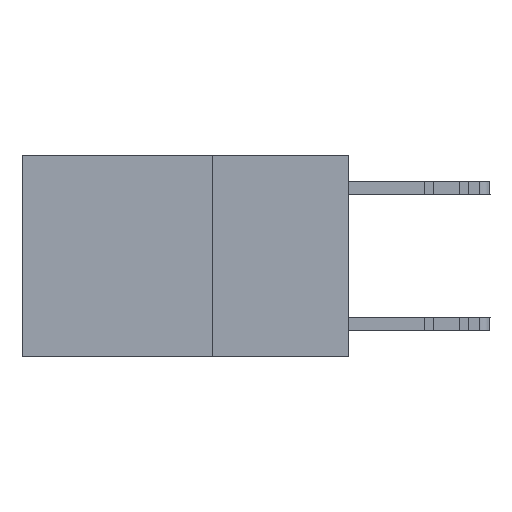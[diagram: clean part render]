
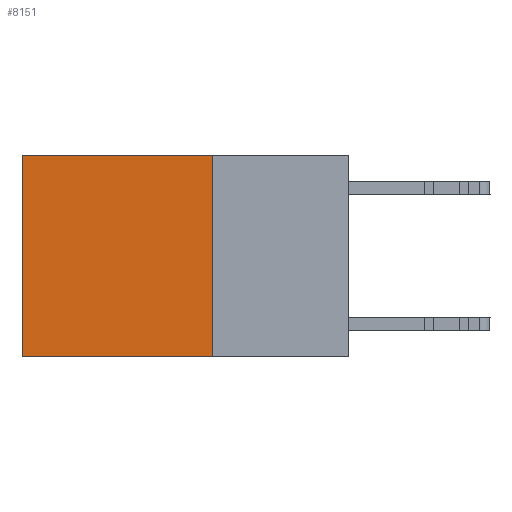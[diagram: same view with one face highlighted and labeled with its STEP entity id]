
A CAD part, left-side view. The second image highlights one B-rep face of the part: STEP entity #8151.
In plain terms, the highlighted planar face has unit normal (-1, 0, 0).
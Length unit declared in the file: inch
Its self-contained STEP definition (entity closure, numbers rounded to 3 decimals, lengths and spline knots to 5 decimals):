
#468 = ORIENTED_EDGE ( 'NONE', *, *, #17017, .T. ) ;
#473 = VECTOR ( 'NONE', #4716, 39.37008 ) ;
#1434 = LINE ( 'NONE', #5708, #473 ) ;
#2839 = CARTESIAN_POINT ( 'NONE',  ( 0.2625, 0.25, 0. ) ) ;
#3138 = DIRECTION ( 'NONE',  ( 0., 0., -1. ) ) ;
#3857 = VERTEX_POINT ( 'NONE', #8000 ) ;
#3904 = EDGE_CURVE ( 'NONE', #3857, #25204, #1434, .T. ) ;
#4211 = EDGE_LOOP ( 'NONE', ( #19752, #15966, #17215, #468 ) ) ;
#4716 = DIRECTION ( 'NONE',  ( 0., 0., -1. ) ) ;
#5372 = DIRECTION ( 'NONE',  ( 0., 0., -1. ) ) ;
#5417 = DIRECTION ( 'NONE',  ( 1., 0., 0. ) ) ;
#5456 = AXIS2_PLACEMENT_3D ( 'NONE', #6065, #5417, #5372 ) ;
#5487 = CARTESIAN_POINT ( 'NONE',  ( 0.2625, 0.25, 0. ) ) ;
#5708 = CARTESIAN_POINT ( 'NONE',  ( 0.2625, 0.6, 0. ) ) ;
#5803 = PLANE ( 'NONE',  #5456 ) ;
#5851 = VERTEX_POINT ( 'NONE', #13735 ) ;
#6065 = CARTESIAN_POINT ( 'NONE',  ( 0.2625, 0.25, 0. ) ) ;
#6564 = EDGE_CURVE ( 'NONE', #15828, #5851, #12730, .T. ) ;
#6654 = CARTESIAN_POINT ( 'NONE',  ( 0.2625, 0.25, -0.37 ) ) ;
#6676 = DIRECTION ( 'NONE',  ( 0., 1., 0. ) ) ;
#8000 = CARTESIAN_POINT ( 'NONE',  ( 0.2625, 0.6, 0. ) ) ;
#8151 = ADVANCED_FACE ( 'NONE', ( #30001 ), #5803, .F. ) ;
#9547 = LINE ( 'NONE', #6654, #9790 ) ;
#9790 = VECTOR ( 'NONE', #6676, 39.37008 ) ;
#9975 = CARTESIAN_POINT ( 'NONE',  ( 0.2625, 0.6, -0.37 ) ) ;
#10419 = EDGE_CURVE ( 'NONE', #5851, #25204, #9547, .T. ) ;
#12532 = VECTOR ( 'NONE', #3138, 39.37008 ) ;
#12730 = LINE ( 'NONE', #2839, #12532 ) ;
#13735 = CARTESIAN_POINT ( 'NONE',  ( 0.2625, 0.25, -0.37 ) ) ;
#15828 = VERTEX_POINT ( 'NONE', #5487 ) ;
#15966 = ORIENTED_EDGE ( 'NONE', *, *, #10419, .F. ) ;
#17017 = EDGE_CURVE ( 'NONE', #15828, #3857, #20449, .T. ) ;
#17215 = ORIENTED_EDGE ( 'NONE', *, *, #6564, .F. ) ;
#19752 = ORIENTED_EDGE ( 'NONE', *, *, #3904, .T. ) ;
#20321 = VECTOR ( 'NONE', #25144, 39.37008 ) ;
#20449 = LINE ( 'NONE', #25277, #20321 ) ;
#25144 = DIRECTION ( 'NONE',  ( 0., 1., 0. ) ) ;
#25204 = VERTEX_POINT ( 'NONE', #9975 ) ;
#25277 = CARTESIAN_POINT ( 'NONE',  ( 0.2625, 0.25, 0. ) ) ;
#30001 = FACE_OUTER_BOUND ( 'NONE', #4211, .T. ) ;
